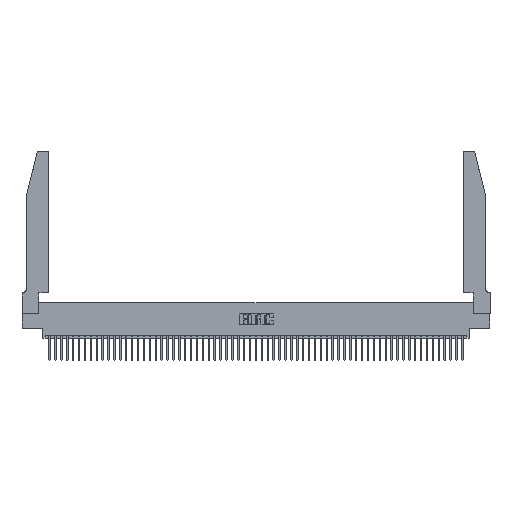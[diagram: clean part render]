
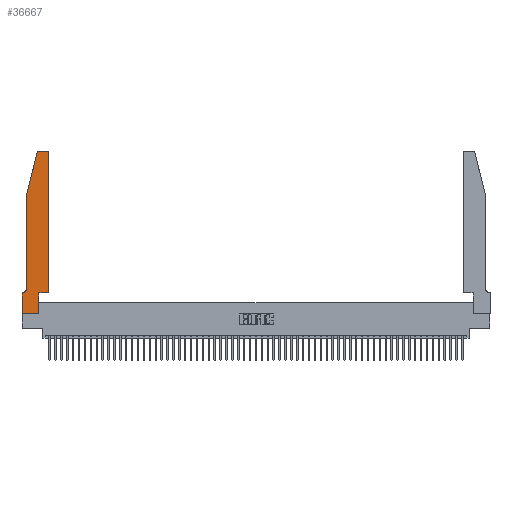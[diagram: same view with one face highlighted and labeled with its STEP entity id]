
A CAD part, top view. The second image highlights one B-rep face of the part: STEP entity #36667.
In plain terms, the highlighted planar face has unit normal (0, 0, 1).
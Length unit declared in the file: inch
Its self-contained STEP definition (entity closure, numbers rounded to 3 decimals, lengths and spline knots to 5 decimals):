
#829 = VECTOR ( 'NONE', #29004, 39.37008 ) ;
#1427 = PLANE ( 'NONE',  #6125 ) ;
#1534 = CARTESIAN_POINT ( 'NONE',  ( 0.4505, 0.35, 0.37 ) ) ;
#1656 = VERTEX_POINT ( 'NONE', #55004 ) ;
#2173 = EDGE_CURVE ( 'NONE', #1656, #11324, #29022, .T. ) ;
#2677 = CARTESIAN_POINT ( 'NONE',  ( 0.0755, 2., 0.37 ) ) ;
#2828 = EDGE_CURVE ( 'NONE', #36451, #17775, #50146, .T. ) ;
#3149 = EDGE_CURVE ( 'NONE', #53905, #51884, #23402, .T. ) ;
#4026 = EDGE_CURVE ( 'NONE', #26498, #1656, #13826, .T. ) ;
#5865 = VERTEX_POINT ( 'NONE', #7403 ) ;
#5892 = DIRECTION ( 'NONE',  ( 0., 0., 1. ) ) ;
#6125 = AXIS2_PLACEMENT_3D ( 'NONE', #32174, #5892, #36604 ) ;
#7077 = CARTESIAN_POINT ( 'NONE',  ( 0., 0., 0.37 ) ) ;
#7379 = CARTESIAN_POINT ( 'NONE',  ( 0.0755, 2., 0.37 ) ) ;
#7403 = CARTESIAN_POINT ( 'NONE',  ( 0., 0., 0.37 ) ) ;
#7513 = VERTEX_POINT ( 'NONE', #32391 ) ;
#7869 = VECTOR ( 'NONE', #24826, 39.37008 ) ;
#7984 = CARTESIAN_POINT ( 'NONE',  ( 0.4205, 2.72, 0.37 ) ) ;
#8402 = ORIENTED_EDGE ( 'NONE', *, *, #14082, .T. ) ;
#8418 = EDGE_CURVE ( 'NONE', #7513, #27790, #22969, .T. ) ;
#8836 = CARTESIAN_POINT ( 'NONE',  ( 0.4205, 2.75, 0.37 ) ) ;
#8975 = VECTOR ( 'NONE', #47824, 39.37008 ) ;
#9074 = ORIENTED_EDGE ( 'NONE', *, *, #25275, .T. ) ;
#9559 = LINE ( 'NONE', #12804, #8975 ) ;
#10381 = EDGE_CURVE ( 'NONE', #51884, #20079, #47506, .T. ) ;
#11126 = CARTESIAN_POINT ( 'NONE',  ( 0.4505, 0.35, 0.37 ) ) ;
#11175 = DIRECTION ( 'NONE',  ( 0., 0., -1. ) ) ;
#11324 = VERTEX_POINT ( 'NONE', #1534 ) ;
#11510 = DIRECTION ( 'NONE',  ( 1., 0., 0. ) ) ;
#12442 = DIRECTION ( 'NONE',  ( 1., 0., 0. ) ) ;
#12804 = CARTESIAN_POINT ( 'NONE',  ( 0.2605, 2.75, 0.37 ) ) ;
#13826 = LINE ( 'NONE', #43153, #47391 ) ;
#14082 = EDGE_CURVE ( 'NONE', #48696, #5865, #51771, .T. ) ;
#14625 = VECTOR ( 'NONE', #51897, 39.37008 ) ;
#15266 = EDGE_CURVE ( 'NONE', #11324, #36451, #18180, .T. ) ;
#16075 = ORIENTED_EDGE ( 'NONE', *, *, #2828, .T. ) ;
#16816 = VECTOR ( 'NONE', #19956, 39.37008 ) ;
#16914 = CARTESIAN_POINT ( 'NONE',  ( 0.4505, 0.35, 0.37 ) ) ;
#17775 = VERTEX_POINT ( 'NONE', #8836 ) ;
#18180 = LINE ( 'NONE', #11126, #16816 ) ;
#19364 = ORIENTED_EDGE ( 'NONE', *, *, #10381, .T. ) ;
#19678 = CARTESIAN_POINT ( 'NONE',  ( 0.284, 2.72, 0.37 ) ) ;
#19956 = DIRECTION ( 'NONE',  ( 0., 1., 0. ) ) ;
#20079 = VERTEX_POINT ( 'NONE', #46562 ) ;
#20131 = ORIENTED_EDGE ( 'NONE', *, *, #29016, .T. ) ;
#21095 = CARTESIAN_POINT ( 'NONE',  ( 0.4505, 2.72, 0.37 ) ) ;
#21148 = DIRECTION ( 'NONE',  ( 0., 1., 0. ) ) ;
#22969 = CIRCLE ( 'NONE', #56341, 0.07 ) ;
#23402 = CIRCLE ( 'NONE', #49284, 0.03 ) ;
#23475 = ORIENTED_EDGE ( 'NONE', *, *, #8418, .T. ) ;
#24069 = DIRECTION ( 'NONE',  ( 1., 0., 0. ) ) ;
#24826 = DIRECTION ( 'NONE',  ( 0., -1., 0. ) ) ;
#25244 = DIRECTION ( 'NONE',  ( 0., -1., 0. ) ) ;
#25275 = EDGE_CURVE ( 'NONE', #20079, #7513, #42858, .T. ) ;
#26394 = CARTESIAN_POINT ( 'NONE',  ( 0.0755, 0.35, 0.37 ) ) ;
#26498 = VERTEX_POINT ( 'NONE', #45478 ) ;
#27790 = VERTEX_POINT ( 'NONE', #45528 ) ;
#28395 = ORIENTED_EDGE ( 'NONE', *, *, #2173, .T. ) ;
#28823 = FACE_OUTER_BOUND ( 'NONE', #45647, .T. ) ;
#29004 = DIRECTION ( 'NONE',  ( -0.239, -0.971, 0. ) ) ;
#29016 = EDGE_CURVE ( 'NONE', #5865, #26498, #33215, .T. ) ;
#29022 = LINE ( 'NONE', #16914, #14625 ) ;
#30535 = ORIENTED_EDGE ( 'NONE', *, *, #3149, .T. ) ;
#32174 = CARTESIAN_POINT ( 'NONE',  ( 0., 0.35, 0.37 ) ) ;
#32391 = CARTESIAN_POINT ( 'NONE',  ( 0.0755, 0.42, 0.37 ) ) ;
#32521 = ORIENTED_EDGE ( 'NONE', *, *, #15266, .T. ) ;
#33215 = LINE ( 'NONE', #7077, #54998 ) ;
#33491 = CARTESIAN_POINT ( 'NONE',  ( 0.284, 2.75, 0.37 ) ) ;
#34406 = VECTOR ( 'NONE', #44036, 39.37008 ) ;
#36451 = VERTEX_POINT ( 'NONE', #21095 ) ;
#36604 = DIRECTION ( 'NONE',  ( 1., 0., 0. ) ) ;
#36667 = ADVANCED_FACE ( 'NONE', ( #28823 ), #1427, .T. ) ;
#37087 = EDGE_CURVE ( 'NONE', #17775, #53905, #9559, .T. ) ;
#37336 = CARTESIAN_POINT ( 'NONE',  ( 0., 0.35, 0.37 ) ) ;
#37453 = CARTESIAN_POINT ( 'NONE',  ( 0.0055, 0.42, 0.37 ) ) ;
#38280 = CARTESIAN_POINT ( 'NONE',  ( 0., 0., 0.37 ) ) ;
#38681 = DIRECTION ( 'NONE',  ( 0., 0., 1. ) ) ;
#41809 = DIRECTION ( 'NONE',  ( -1., 0., 0. ) ) ;
#42858 = LINE ( 'NONE', #7379, #7869 ) ;
#43153 = CARTESIAN_POINT ( 'NONE',  ( 0.2865, 0.35, 0.37 ) ) ;
#44036 = DIRECTION ( 'NONE',  ( -1., 0., 0. ) ) ;
#45478 = CARTESIAN_POINT ( 'NONE',  ( 0.2865, 0., 0.37 ) ) ;
#45528 = CARTESIAN_POINT ( 'NONE',  ( 0.0055, 0.35, 0.37 ) ) ;
#45647 = EDGE_LOOP ( 'NONE', ( #50733, #30535, #19364, #9074, #23475, #50876, #8402, #20131, #46198, #28395, #32521, #16075 ) ) ;
#46030 = LINE ( 'NONE', #26394, #34406 ) ;
#46198 = ORIENTED_EDGE ( 'NONE', *, *, #4026, .T. ) ;
#46226 = CARTESIAN_POINT ( 'NONE',  ( 0.25487, 2.72718, 0.37 ) ) ;
#46562 = CARTESIAN_POINT ( 'NONE',  ( 0.0755, 2., 0.37 ) ) ;
#47391 = VECTOR ( 'NONE', #21148, 39.37008 ) ;
#47506 = LINE ( 'NONE', #2677, #829 ) ;
#47824 = DIRECTION ( 'NONE',  ( -1., 0., 0. ) ) ;
#48696 = VERTEX_POINT ( 'NONE', #37336 ) ;
#49284 = AXIS2_PLACEMENT_3D ( 'NONE', #19678, #50297, #24069 ) ;
#50146 = CIRCLE ( 'NONE', #50364, 0.03 ) ;
#50297 = DIRECTION ( 'NONE',  ( 0., 0., 1. ) ) ;
#50364 = AXIS2_PLACEMENT_3D ( 'NONE', #7984, #38681, #12442 ) ;
#50394 = VECTOR ( 'NONE', #25244, 39.37008 ) ;
#50733 = ORIENTED_EDGE ( 'NONE', *, *, #37087, .T. ) ;
#50876 = ORIENTED_EDGE ( 'NONE', *, *, #53530, .T. ) ;
#51771 = LINE ( 'NONE', #38280, #50394 ) ;
#51884 = VERTEX_POINT ( 'NONE', #46226 ) ;
#51897 = DIRECTION ( 'NONE',  ( 1., 0., 0. ) ) ;
#53530 = EDGE_CURVE ( 'NONE', #27790, #48696, #46030, .T. ) ;
#53905 = VERTEX_POINT ( 'NONE', #33491 ) ;
#54998 = VECTOR ( 'NONE', #11510, 39.37008 ) ;
#55004 = CARTESIAN_POINT ( 'NONE',  ( 0.2865, 0.35, 0.37 ) ) ;
#56341 = AXIS2_PLACEMENT_3D ( 'NONE', #37453, #11175, #41809 ) ;
